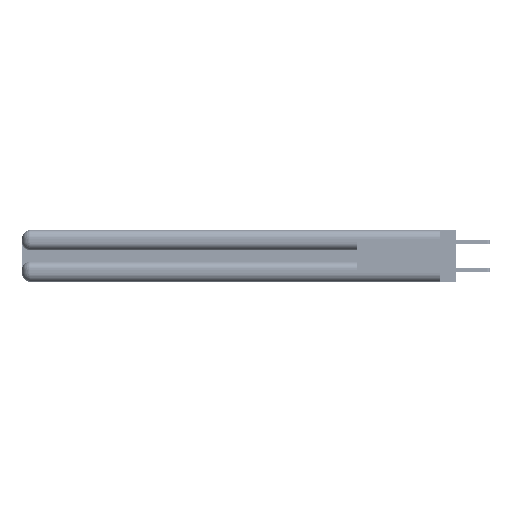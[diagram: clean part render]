
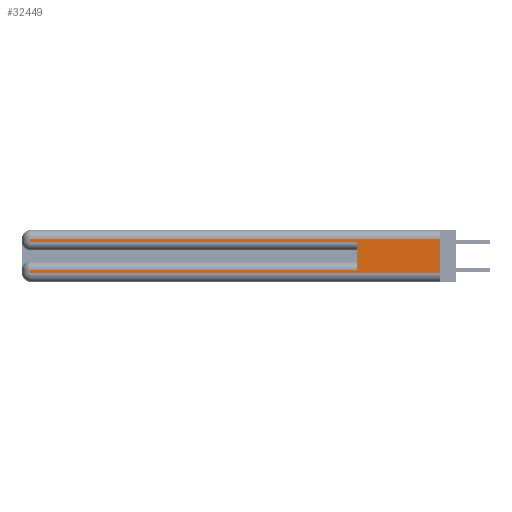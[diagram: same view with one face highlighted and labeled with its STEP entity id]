
A CAD part, left-side view. The second image highlights one B-rep face of the part: STEP entity #32449.
In plain terms, the highlighted planar face has unit normal (-1, 0, 0).
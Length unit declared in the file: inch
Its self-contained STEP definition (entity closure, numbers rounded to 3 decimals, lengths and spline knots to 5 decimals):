
#961 = CARTESIAN_POINT ( 'NONE',  ( 0., 0., 0.06 ) ) ;
#1059 = CARTESIAN_POINT ( 'NONE',  ( 0., 0., 0.285 ) ) ;
#1096 = VERTEX_POINT ( 'NONE', #961 ) ;
#1586 = CARTESIAN_POINT ( 'NONE',  ( 0., 0.6, 0.145 ) ) ;
#2319 = VECTOR ( 'NONE', #13463, 39.37008 ) ;
#2413 = VERTEX_POINT ( 'NONE', #38055 ) ;
#3996 = CARTESIAN_POINT ( 'NONE',  ( 0., 0., 0.37 ) ) ;
#4836 = VERTEX_POINT ( 'NONE', #35957 ) ;
#5065 = VECTOR ( 'NONE', #49622, 39.37008 ) ;
#5510 = VERTEX_POINT ( 'NONE', #44516 ) ;
#5852 = EDGE_CURVE ( 'NONE', #4836, #1096, #33188, .T. ) ;
#6515 = VECTOR ( 'NONE', #21611, 39.37008 ) ;
#6542 = EDGE_CURVE ( 'NONE', #35970, #13054, #36809, .T. ) ;
#7800 = DIRECTION ( 'NONE',  ( 0., 0., -1. ) ) ;
#7828 = VECTOR ( 'NONE', #24708, 39.37008 ) ;
#8120 = CARTESIAN_POINT ( 'NONE',  ( 0., 2.94, 0.37 ) ) ;
#11521 = VECTOR ( 'NONE', #35964, 39.37008 ) ;
#12588 = CARTESIAN_POINT ( 'NONE',  ( 0., 0., 0.31 ) ) ;
#13054 = VERTEX_POINT ( 'NONE', #20274 ) ;
#13239 = EDGE_CURVE ( 'NONE', #39308, #1096, #45490, .T. ) ;
#13463 = DIRECTION ( 'NONE',  ( 0., -1., 0. ) ) ;
#18246 = CARTESIAN_POINT ( 'NONE',  ( 0., 0., 0.085 ) ) ;
#18623 = EDGE_CURVE ( 'NONE', #42116, #2413, #42842, .T. ) ;
#19704 = ORIENTED_EDGE ( 'NONE', *, *, #45220, .T. ) ;
#20274 = CARTESIAN_POINT ( 'NONE',  ( 0., 2.94, 0.285 ) ) ;
#20685 = CARTESIAN_POINT ( 'NONE',  ( 0., 2.94, 0.37 ) ) ;
#20821 = LINE ( 'NONE', #1059, #2319 ) ;
#21306 = DIRECTION ( 'NONE',  ( 0., 0., -1. ) ) ;
#21611 = DIRECTION ( 'NONE',  ( 0., -1., 0. ) ) ;
#23244 = LINE ( 'NONE', #12588, #11521 ) ;
#23704 = DIRECTION ( 'NONE',  ( 1., 0., 0. ) ) ;
#23915 = LINE ( 'NONE', #20685, #7828 ) ;
#24708 = DIRECTION ( 'NONE',  ( 0., 0., -1. ) ) ;
#24785 = ORIENTED_EDGE ( 'NONE', *, *, #18623, .F. ) ;
#27173 = ORIENTED_EDGE ( 'NONE', *, *, #33364, .T. ) ;
#29954 = CARTESIAN_POINT ( 'NONE',  ( 0., 2.94, 0.31 ) ) ;
#31518 = FACE_OUTER_BOUND ( 'NONE', #47168, .T. ) ;
#31713 = CARTESIAN_POINT ( 'NONE',  ( 0., 0., 0.06 ) ) ;
#31824 = VECTOR ( 'NONE', #21306, 39.37008 ) ;
#32449 = ADVANCED_FACE ( 'NONE', ( #31518 ), #39358, .F. ) ;
#33188 = LINE ( 'NONE', #31713, #6515 ) ;
#33364 = EDGE_CURVE ( 'NONE', #5510, #4836, #23915, .T. ) ;
#33517 = VECTOR ( 'NONE', #40894, 39.37008 ) ;
#33839 = ORIENTED_EDGE ( 'NONE', *, *, #13239, .F. ) ;
#35957 = CARTESIAN_POINT ( 'NONE',  ( 0., 2.94, 0.06 ) ) ;
#35964 = DIRECTION ( 'NONE',  ( 0., 1., 0. ) ) ;
#35970 = VERTEX_POINT ( 'NONE', #29954 ) ;
#36056 = ORIENTED_EDGE ( 'NONE', *, *, #5852, .T. ) ;
#36809 = LINE ( 'NONE', #8120, #49789 ) ;
#37538 = ORIENTED_EDGE ( 'NONE', *, *, #42145, .T. ) ;
#38055 = CARTESIAN_POINT ( 'NONE',  ( 0., 0.6, 0.285 ) ) ;
#39308 = VERTEX_POINT ( 'NONE', #46226 ) ;
#39358 = PLANE ( 'NONE',  #51137 ) ;
#39664 = CARTESIAN_POINT ( 'NONE',  ( 0., 0.6, 0.085 ) ) ;
#40372 = ORIENTED_EDGE ( 'NONE', *, *, #6542, .T. ) ;
#40894 = DIRECTION ( 'NONE',  ( 0., 0., 1. ) ) ;
#41028 = LINE ( 'NONE', #18246, #5065 ) ;
#42116 = VERTEX_POINT ( 'NONE', #39664 ) ;
#42145 = EDGE_CURVE ( 'NONE', #13054, #2413, #20821, .T. ) ;
#42842 = LINE ( 'NONE', #1586, #33517 ) ;
#44516 = CARTESIAN_POINT ( 'NONE',  ( 0., 2.94, 0.085 ) ) ;
#44776 = CARTESIAN_POINT ( 'NONE',  ( 0., 0., 0.37 ) ) ;
#45220 = EDGE_CURVE ( 'NONE', #42116, #5510, #41028, .T. ) ;
#45490 = LINE ( 'NONE', #44776, #31824 ) ;
#46226 = CARTESIAN_POINT ( 'NONE',  ( 0., 0., 0.31 ) ) ;
#47168 = EDGE_LOOP ( 'NONE', ( #33839, #49327, #40372, #37538, #24785, #19704, #27173, #36056 ) ) ;
#49327 = ORIENTED_EDGE ( 'NONE', *, *, #50205, .T. ) ;
#49622 = DIRECTION ( 'NONE',  ( 0., 1., 0. ) ) ;
#49789 = VECTOR ( 'NONE', #50548, 39.37008 ) ;
#50205 = EDGE_CURVE ( 'NONE', #39308, #35970, #23244, .T. ) ;
#50548 = DIRECTION ( 'NONE',  ( 0., 0., -1. ) ) ;
#51137 = AXIS2_PLACEMENT_3D ( 'NONE', #3996, #23704, #7800 ) ;
